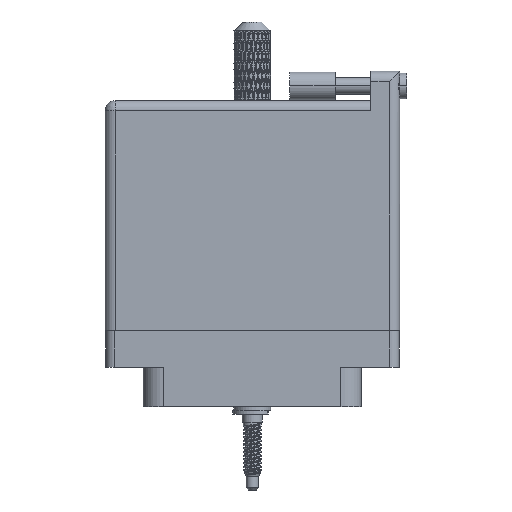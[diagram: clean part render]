
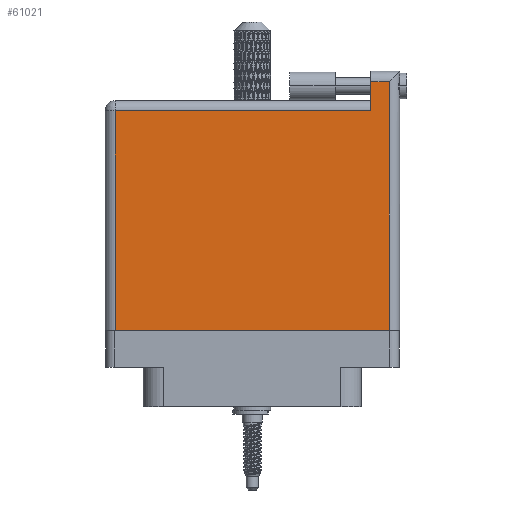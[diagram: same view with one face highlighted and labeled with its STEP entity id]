
A CAD part, front view. The second image highlights one B-rep face of the part: STEP entity #61021.
In plain terms, the highlighted face is planar.
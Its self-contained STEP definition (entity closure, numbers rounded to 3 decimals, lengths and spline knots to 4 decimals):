
#1140 = VERTEX_POINT ( 'NONE', #5433 ) ;
#2811 = DIRECTION ( 'NONE',  ( 0., -1., 0. ) ) ;
#4568 = ORIENTED_EDGE ( 'NONE', *, *, #85889, .T. ) ;
#5433 = CARTESIAN_POINT ( 'NONE',  ( -0.934, 1.396, 0.4495 ) ) ;
#8013 = CARTESIAN_POINT ( 'NONE',  ( 0.934, -0.1, 0.4495 ) ) ;
#8707 = VERTEX_POINT ( 'NONE', #39353 ) ;
#9478 = VECTOR ( 'NONE', #36531, 39.3701 ) ;
#10237 = FACE_OUTER_BOUND ( 'NONE', #19762, .T. ) ;
#10599 = CARTESIAN_POINT ( 'NONE',  ( -1.004, 1.596, 0.4495 ) ) ;
#12463 = AXIS2_PLACEMENT_3D ( 'NONE', #95687, #46890, #71461 ) ;
#14607 = CARTESIAN_POINT ( 'NONE',  ( -1.004, 1.396, 0.4495 ) ) ;
#14749 = CARTESIAN_POINT ( 'NONE',  ( 0.807, 1.596, 0.4495 ) ) ;
#17780 = CARTESIAN_POINT ( 'NONE',  ( -0.934, -0.1, 0.4495 ) ) ;
#19762 = EDGE_LOOP ( 'NONE', ( #47738, #4568, #49856, #62299, #66727, #70998 ) ) ;
#20205 = CARTESIAN_POINT ( 'NONE',  ( -1.004, -0.1, 0.4495 ) ) ;
#26936 = EDGE_CURVE ( 'NONE', #82101, #8707, #53248, .T. ) ;
#31528 = DIRECTION ( 'NONE',  ( 0., 1., 0. ) ) ;
#31785 = CARTESIAN_POINT ( 'NONE',  ( 0.934, 1.596, 0.4495 ) ) ;
#33285 = VECTOR ( 'NONE', #70856, 39.3701 ) ;
#36531 = DIRECTION ( 'NONE',  ( 1., 0., 0. ) ) ;
#38681 = PLANE ( 'NONE',  #12463 ) ;
#39097 = CARTESIAN_POINT ( 'NONE',  ( 0.807, 1.666, 0.4495 ) ) ;
#39353 = CARTESIAN_POINT ( 'NONE',  ( 0.807, 1.396, 0.4495 ) ) ;
#40218 = LINE ( 'NONE', #17780, #84840 ) ;
#44347 = VECTOR ( 'NONE', #72580, 39.3701 ) ;
#46890 = DIRECTION ( 'NONE',  ( 0., 0., -1. ) ) ;
#47738 = ORIENTED_EDGE ( 'NONE', *, *, #81116, .T. ) ;
#48139 = EDGE_CURVE ( 'NONE', #87121, #82101, #83439, .T. ) ;
#49028 = LINE ( 'NONE', #20205, #9478 ) ;
#49856 = ORIENTED_EDGE ( 'NONE', *, *, #48139, .T. ) ;
#50391 = EDGE_CURVE ( 'NONE', #8707, #1140, #60155, .T. ) ;
#52943 = DIRECTION ( 'NONE',  ( -1., 0., 0. ) ) ;
#53248 = LINE ( 'NONE', #39097, #44347 ) ;
#59937 = VERTEX_POINT ( 'NONE', #8013 ) ;
#60155 = LINE ( 'NONE', #14607, #33285 ) ;
#61021 = ADVANCED_FACE ( 'NONE', ( #10237 ), #38681, .F. ) ;
#62299 = ORIENTED_EDGE ( 'NONE', *, *, #26936, .T. ) ;
#66727 = ORIENTED_EDGE ( 'NONE', *, *, #50391, .T. ) ;
#67749 = EDGE_CURVE ( 'NONE', #1140, #77296, #40218, .T. ) ;
#70856 = DIRECTION ( 'NONE',  ( -1., 0., 0. ) ) ;
#70998 = ORIENTED_EDGE ( 'NONE', *, *, #67749, .T. ) ;
#71461 = DIRECTION ( 'NONE',  ( -1., 0., 0. ) ) ;
#72580 = DIRECTION ( 'NONE',  ( 0., -1., 0. ) ) ;
#75123 = VECTOR ( 'NONE', #31528, 39.3701 ) ;
#77069 = VECTOR ( 'NONE', #52943, 39.3701 ) ;
#77296 = VERTEX_POINT ( 'NONE', #104710 ) ;
#77677 = LINE ( 'NONE', #105381, #75123 ) ;
#81116 = EDGE_CURVE ( 'NONE', #77296, #59937, #49028, .T. ) ;
#82101 = VERTEX_POINT ( 'NONE', #14749 ) ;
#83439 = LINE ( 'NONE', #10599, #77069 ) ;
#84840 = VECTOR ( 'NONE', #2811, 39.3701 ) ;
#85889 = EDGE_CURVE ( 'NONE', #59937, #87121, #77677, .T. ) ;
#87121 = VERTEX_POINT ( 'NONE', #31785 ) ;
#95687 = CARTESIAN_POINT ( 'NONE',  ( -1.004, 1.466, 0.4495 ) ) ;
#104710 = CARTESIAN_POINT ( 'NONE',  ( -0.934, -0.1, 0.4495 ) ) ;
#105381 = CARTESIAN_POINT ( 'NONE',  ( 0.934, 1.666, 0.4495 ) ) ;
